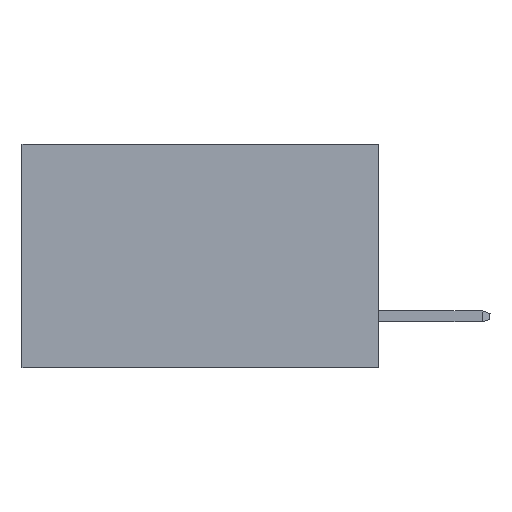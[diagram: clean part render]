
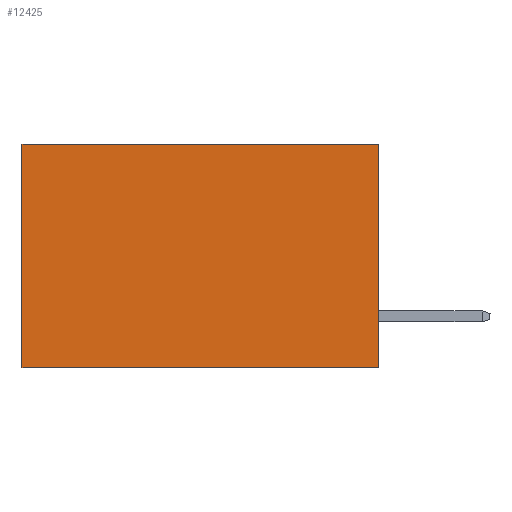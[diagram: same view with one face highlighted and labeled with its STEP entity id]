
A CAD part, left-side view. The second image highlights one B-rep face of the part: STEP entity #12425.
In plain terms, the highlighted planar face has unit normal (-1, 0, 0).
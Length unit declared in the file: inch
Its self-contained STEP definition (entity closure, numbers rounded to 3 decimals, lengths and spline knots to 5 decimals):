
#1064 = CARTESIAN_POINT ( 'NONE',  ( 0.277, 0., -0.37 ) ) ;
#1155 = CARTESIAN_POINT ( 'NONE',  ( 0.277, 0.59, 0. ) ) ;
#1508 = EDGE_CURVE ( 'NONE', #17783, #12150, #7111, .T. ) ;
#1930 = VERTEX_POINT ( 'NONE', #1155 ) ;
#3172 = EDGE_CURVE ( 'NONE', #1930, #5974, #21055, .T. ) ;
#3683 = LINE ( 'NONE', #4821, #16597 ) ;
#4821 = CARTESIAN_POINT ( 'NONE',  ( 0.277, 0., -0.37 ) ) ;
#5124 = EDGE_CURVE ( 'NONE', #17783, #1930, #16915, .T. ) ;
#5974 = VERTEX_POINT ( 'NONE', #6460 ) ;
#6460 = CARTESIAN_POINT ( 'NONE',  ( 0.277, 0.59, -0.37 ) ) ;
#6552 = DIRECTION ( 'NONE',  ( 0., 1., 0. ) ) ;
#6649 = CARTESIAN_POINT ( 'NONE',  ( 0.277, 0., 0. ) ) ;
#6981 = DIRECTION ( 'NONE',  ( 0., 0., -1. ) ) ;
#7111 = LINE ( 'NONE', #1064, #16531 ) ;
#7309 = VECTOR ( 'NONE', #6981, 39.37008 ) ;
#10602 = PLANE ( 'NONE',  #18742 ) ;
#10680 = CARTESIAN_POINT ( 'NONE',  ( 0.277, 0., -0.37 ) ) ;
#11218 = FACE_OUTER_BOUND ( 'NONE', #21164, .T. ) ;
#11677 = ORIENTED_EDGE ( 'NONE', *, *, #3172, .T. ) ;
#12150 = VERTEX_POINT ( 'NONE', #17220 ) ;
#12425 = ADVANCED_FACE ( 'NONE', ( #11218 ), #10602, .F. ) ;
#12551 = ORIENTED_EDGE ( 'NONE', *, *, #18050, .F. ) ;
#13347 = ORIENTED_EDGE ( 'NONE', *, *, #1508, .F. ) ;
#13365 = ORIENTED_EDGE ( 'NONE', *, *, #5124, .T. ) ;
#13669 = DIRECTION ( 'NONE',  ( 0., 0., -1. ) ) ;
#13805 = DIRECTION ( 'NONE',  ( 1., 0., 0. ) ) ;
#15453 = DIRECTION ( 'NONE',  ( 0., 1., 0. ) ) ;
#15544 = CARTESIAN_POINT ( 'NONE',  ( 0.277, 0., 0. ) ) ;
#15751 = DIRECTION ( 'NONE',  ( 0., 0., -1. ) ) ;
#16531 = VECTOR ( 'NONE', #15751, 39.37008 ) ;
#16597 = VECTOR ( 'NONE', #6552, 39.37008 ) ;
#16915 = LINE ( 'NONE', #15544, #20695 ) ;
#17220 = CARTESIAN_POINT ( 'NONE',  ( 0.277, 0., -0.37 ) ) ;
#17783 = VERTEX_POINT ( 'NONE', #6649 ) ;
#18050 = EDGE_CURVE ( 'NONE', #12150, #5974, #3683, .T. ) ;
#18742 = AXIS2_PLACEMENT_3D ( 'NONE', #10680, #13805, #13669 ) ;
#19978 = CARTESIAN_POINT ( 'NONE',  ( 0.277, 0.59, -0.37 ) ) ;
#20695 = VECTOR ( 'NONE', #15453, 39.37008 ) ;
#21055 = LINE ( 'NONE', #19978, #7309 ) ;
#21164 = EDGE_LOOP ( 'NONE', ( #11677, #12551, #13347, #13365 ) ) ;
